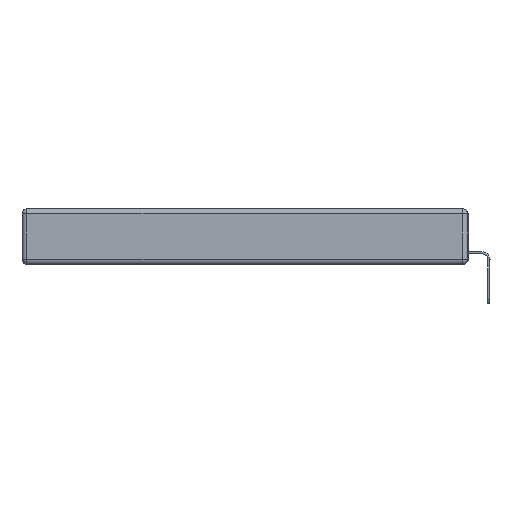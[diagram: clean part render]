
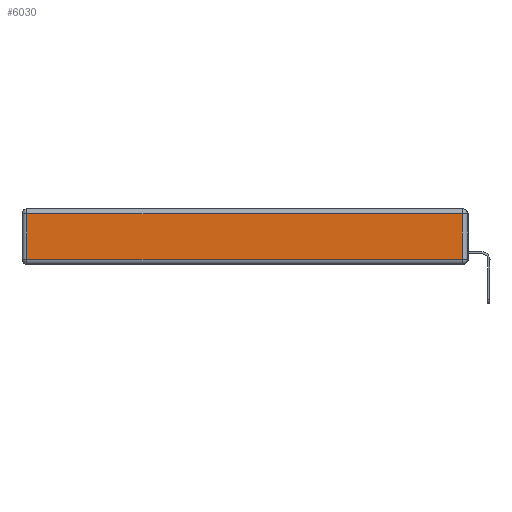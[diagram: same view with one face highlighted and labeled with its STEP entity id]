
A CAD part, left-side view. The second image highlights one B-rep face of the part: STEP entity #6030.
In plain terms, the highlighted planar face has unit normal (-1, 0, 0).
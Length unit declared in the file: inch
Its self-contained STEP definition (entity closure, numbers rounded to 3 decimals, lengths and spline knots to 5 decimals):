
#113 = EDGE_CURVE ( 'NONE', #6726, #1723, #11304, .T. ) ;
#350 = EDGE_CURVE ( 'NONE', #8372, #6726, #12804, .T. ) ;
#357 = VERTEX_POINT ( 'NONE', #15193 ) ;
#999 = DIRECTION ( 'NONE',  ( 0., -1., 0. ) ) ;
#1056 = ORIENTED_EDGE ( 'NONE', *, *, #4739, .T. ) ;
#1104 = VECTOR ( 'NONE', #7888, 39.37008 ) ;
#1235 = CARTESIAN_POINT ( 'NONE',  ( 0., 2.72, -0.343 ) ) ;
#1723 = VERTEX_POINT ( 'NONE', #8960 ) ;
#2115 = CARTESIAN_POINT ( 'NONE',  ( 0., 0.03, -0.343 ) ) ;
#3101 = LINE ( 'NONE', #14129, #13854 ) ;
#3647 = DIRECTION ( 'NONE',  ( 0., 0., -1. ) ) ;
#4411 = DIRECTION ( 'NONE',  ( 0., 0., 1. ) ) ;
#4520 = AXIS2_PLACEMENT_3D ( 'NONE', #15031, #8950, #4411 ) ;
#4737 = CARTESIAN_POINT ( 'NONE',  ( 0., 0.03, -0.313 ) ) ;
#4739 = EDGE_CURVE ( 'NONE', #1723, #357, #13284, .T. ) ;
#5191 = EDGE_LOOP ( 'NONE', ( #11010, #7513, #12297, #1056 ) ) ;
#5349 = CARTESIAN_POINT ( 'NONE',  ( 0., 0.03, -0.03 ) ) ;
#6030 = ADVANCED_FACE ( 'NONE', ( #15281 ), #13740, .T. ) ;
#6101 = DIRECTION ( 'NONE',  ( 0., 1., 0. ) ) ;
#6726 = VERTEX_POINT ( 'NONE', #5349 ) ;
#7513 = ORIENTED_EDGE ( 'NONE', *, *, #350, .T. ) ;
#7888 = DIRECTION ( 'NONE',  ( 0., 0., 1. ) ) ;
#8372 = VERTEX_POINT ( 'NONE', #4737 ) ;
#8521 = CARTESIAN_POINT ( 'NONE',  ( 0., 2.75, -0.03 ) ) ;
#8950 = DIRECTION ( 'NONE',  ( -1., 0., 0. ) ) ;
#8960 = CARTESIAN_POINT ( 'NONE',  ( 0., 2.72, -0.03 ) ) ;
#9458 = VECTOR ( 'NONE', #6101, 39.37008 ) ;
#10171 = EDGE_CURVE ( 'NONE', #357, #8372, #3101, .T. ) ;
#10476 = VECTOR ( 'NONE', #3647, 39.37008 ) ;
#11010 = ORIENTED_EDGE ( 'NONE', *, *, #10171, .T. ) ;
#11304 = LINE ( 'NONE', #8521, #9458 ) ;
#12297 = ORIENTED_EDGE ( 'NONE', *, *, #113, .T. ) ;
#12804 = LINE ( 'NONE', #2115, #1104 ) ;
#13284 = LINE ( 'NONE', #1235, #10476 ) ;
#13740 = PLANE ( 'NONE',  #4520 ) ;
#13854 = VECTOR ( 'NONE', #999, 39.37008 ) ;
#14129 = CARTESIAN_POINT ( 'NONE',  ( 0., 0., -0.313 ) ) ;
#15031 = CARTESIAN_POINT ( 'NONE',  ( 0., 0., -0.343 ) ) ;
#15193 = CARTESIAN_POINT ( 'NONE',  ( 0., 2.72, -0.313 ) ) ;
#15281 = FACE_OUTER_BOUND ( 'NONE', #5191, .T. ) ;
